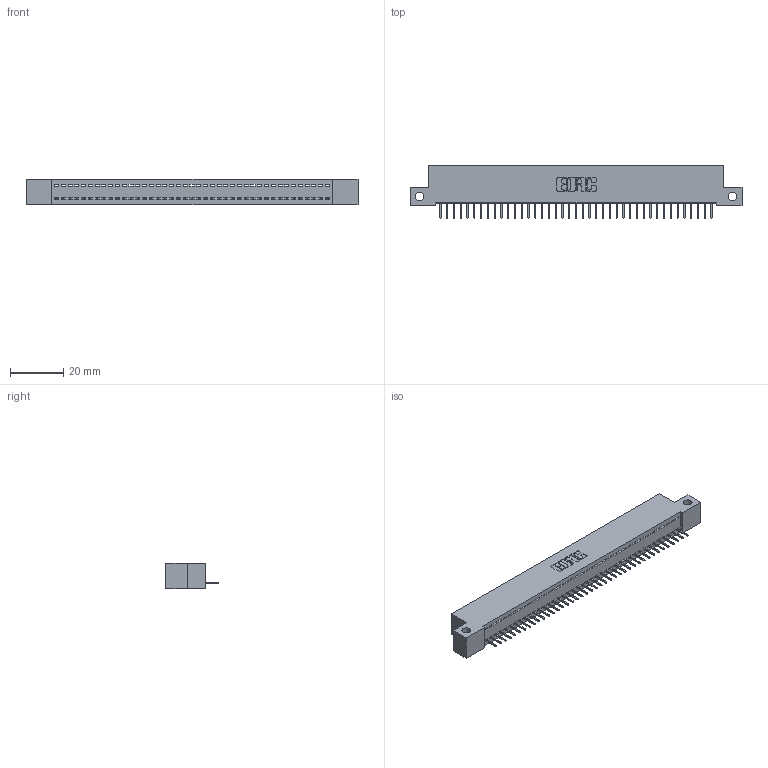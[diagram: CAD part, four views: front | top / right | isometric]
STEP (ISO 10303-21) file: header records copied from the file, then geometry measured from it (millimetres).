
FILE_DESCRIPTION (( 'STEP AP203' ), '1' );
FILE_NAME ('392-041-524-112.STEP', '2019-10-07T20:32:19', ( '' ), ( '' ), 'SwSTEP 2.0', 'SolidWorks 2016', '' );
FILE_SCHEMA (( 'CONFIG_CONTROL_DESIGN' ));
Length unit declared in the file: inch
Products named in the file (3): 342 Part_Side Mount; 345-292-001_345-293-124; 392-041-524-112
Assembly tree (42 placements, depth 2):
  392-041-524-112
    342 Part_Side Mount
    345-292-001_345-293-124  x41
Bounding box: 124.46 x 19.69 x 9.4 mm (x, y, z)
Volume: 10673.1 mm3; surface area: 14988.1 mm2
Topology: 42 solids, 42 shells, 2652 faces, 7679 edges, 4954 vertices
Faces by surface type: plane 2034, cylinder 618
Entity records: 25139 total; most frequent: CARTESIAN_POINT 4341, ORIENTED_EDGE 4318, DIRECTION 3665, EDGE_CURVE 2159, VECTOR 2035, LINE 2035, VERTEX_POINT 1434, AXIS2_PLACEMENT_3D 815
